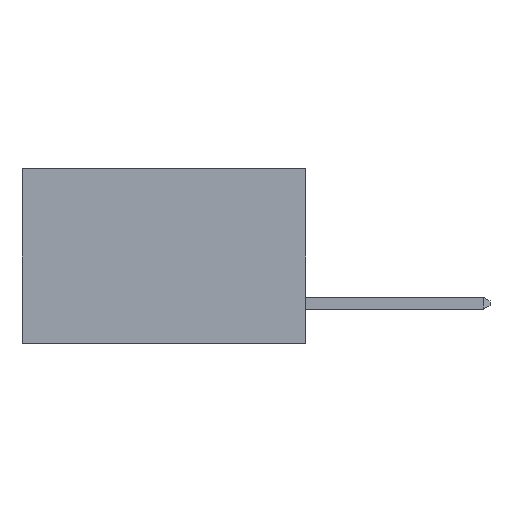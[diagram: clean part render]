
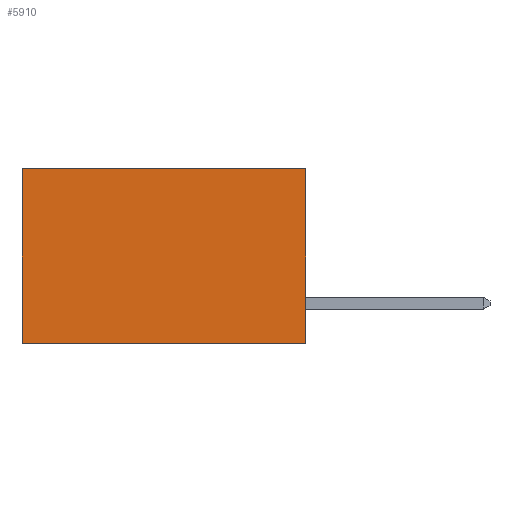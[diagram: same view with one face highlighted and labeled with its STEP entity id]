
A CAD part, left-side view. The second image highlights one B-rep face of the part: STEP entity #5910.
In plain terms, the highlighted planar face has unit normal (-1, 0, 0).
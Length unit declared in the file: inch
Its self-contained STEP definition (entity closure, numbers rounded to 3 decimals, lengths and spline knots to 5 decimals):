
#69 = ORIENTED_EDGE ( 'NONE', *, *, #4165, .T. ) ;
#422 = CARTESIAN_POINT ( 'NONE',  ( 0.2615, 0., -0.37 ) ) ;
#452 = DIRECTION ( 'NONE',  ( 0., 0., -1. ) ) ;
#614 = VERTEX_POINT ( 'NONE', #2262 ) ;
#679 = EDGE_LOOP ( 'NONE', ( #69, #2865, #767, #8479 ) ) ;
#767 = ORIENTED_EDGE ( 'NONE', *, *, #886, .F. ) ;
#886 = EDGE_CURVE ( 'NONE', #614, #5707, #4968, .T. ) ;
#1155 = CARTESIAN_POINT ( 'NONE',  ( 0.2615, 0., -0.37 ) ) ;
#1929 = EDGE_CURVE ( 'NONE', #5707, #8438, #8091, .T. ) ;
#2246 = CARTESIAN_POINT ( 'NONE',  ( 0.2615, 0., 0. ) ) ;
#2262 = CARTESIAN_POINT ( 'NONE',  ( 0.2615, 0., 0. ) ) ;
#2421 = CARTESIAN_POINT ( 'NONE',  ( 0.2615, 0., -0.37 ) ) ;
#2427 = VECTOR ( 'NONE', #6508, 39.37008 ) ;
#2459 = DIRECTION ( 'NONE',  ( 0., 0., -1. ) ) ;
#2865 = ORIENTED_EDGE ( 'NONE', *, *, #1929, .F. ) ;
#3383 = PLANE ( 'NONE',  #4247 ) ;
#4165 = EDGE_CURVE ( 'NONE', #8123, #8438, #6097, .T. ) ;
#4247 = AXIS2_PLACEMENT_3D ( 'NONE', #422, #4758, #452 ) ;
#4311 = LINE ( 'NONE', #2246, #2427 ) ;
#4685 = VECTOR ( 'NONE', #6717, 39.37008 ) ;
#4744 = VECTOR ( 'NONE', #2459, 39.37008 ) ;
#4758 = DIRECTION ( 'NONE',  ( 1., 0., 0. ) ) ;
#4968 = LINE ( 'NONE', #1155, #4744 ) ;
#5011 = EDGE_CURVE ( 'NONE', #614, #8123, #4311, .T. ) ;
#5211 = CARTESIAN_POINT ( 'NONE',  ( 0.2615, 0.6, -0.37 ) ) ;
#5464 = DIRECTION ( 'NONE',  ( 0., 1., 0. ) ) ;
#5707 = VERTEX_POINT ( 'NONE', #2421 ) ;
#5910 = ADVANCED_FACE ( 'NONE', ( #8697 ), #3383, .F. ) ;
#5918 = VECTOR ( 'NONE', #5464, 39.37008 ) ;
#6097 = LINE ( 'NONE', #6753, #4685 ) ;
#6233 = CARTESIAN_POINT ( 'NONE',  ( 0.2615, 0., -0.37 ) ) ;
#6508 = DIRECTION ( 'NONE',  ( 0., 1., 0. ) ) ;
#6717 = DIRECTION ( 'NONE',  ( 0., 0., -1. ) ) ;
#6753 = CARTESIAN_POINT ( 'NONE',  ( 0.2615, 0.6, -0.37 ) ) ;
#8091 = LINE ( 'NONE', #6233, #5918 ) ;
#8123 = VERTEX_POINT ( 'NONE', #8256 ) ;
#8256 = CARTESIAN_POINT ( 'NONE',  ( 0.2615, 0.6, 0. ) ) ;
#8438 = VERTEX_POINT ( 'NONE', #5211 ) ;
#8479 = ORIENTED_EDGE ( 'NONE', *, *, #5011, .T. ) ;
#8697 = FACE_OUTER_BOUND ( 'NONE', #679, .T. ) ;
